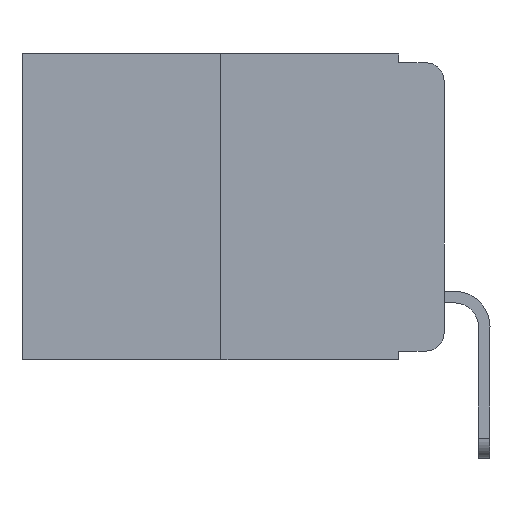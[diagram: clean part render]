
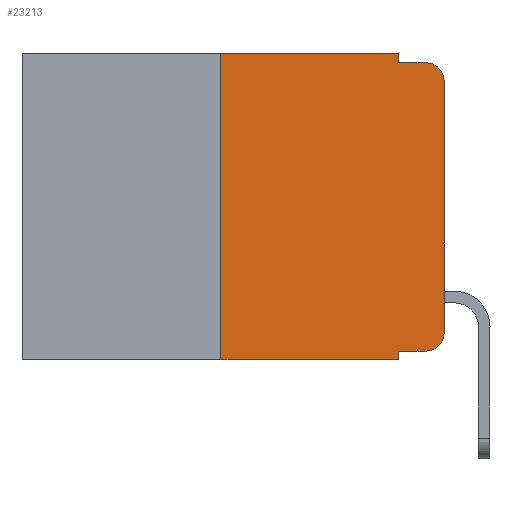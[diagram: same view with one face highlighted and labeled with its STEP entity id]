
A CAD part, left-side view. The second image highlights one B-rep face of the part: STEP entity #23213.
In plain terms, the highlighted planar face has unit normal (-1, 0, 0).
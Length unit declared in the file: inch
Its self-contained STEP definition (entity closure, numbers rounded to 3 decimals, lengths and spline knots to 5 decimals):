
#161 = EDGE_CURVE ( 'NONE', #10687, #3173, #15386, .T. ) ;
#646 = FACE_OUTER_BOUND ( 'NONE', #6226, .T. ) ;
#1108 = EDGE_CURVE ( 'NONE', #1517, #12400, #9660, .T. ) ;
#1128 = VECTOR ( 'NONE', #4296, 39.37008 ) ;
#1149 = CARTESIAN_POINT ( 'NONE',  ( 0., 0.051, -0.343 ) ) ;
#1398 = ORIENTED_EDGE ( 'NONE', *, *, #16433, .F. ) ;
#1502 = VERTEX_POINT ( 'NONE', #22279 ) ;
#1517 = VERTEX_POINT ( 'NONE', #6503 ) ;
#1681 = DIRECTION ( 'NONE',  ( 0., 0., -1. ) ) ;
#1985 = DIRECTION ( 'NONE',  ( -1., 0., 0. ) ) ;
#2085 = VERTEX_POINT ( 'NONE', #11511 ) ;
#2669 = VECTOR ( 'NONE', #2783, 39.37008 ) ;
#2783 = DIRECTION ( 'NONE',  ( 0., -1., 0. ) ) ;
#3173 = VERTEX_POINT ( 'NONE', #8655 ) ;
#3467 = DIRECTION ( 'NONE',  ( -1., 0., 0. ) ) ;
#3740 = DIRECTION ( 'NONE',  ( 0., 0., -1. ) ) ;
#3955 = DIRECTION ( 'NONE',  ( 0., 0., -1. ) ) ;
#4044 = VECTOR ( 'NONE', #16889, 39.37008 ) ;
#4296 = DIRECTION ( 'NONE',  ( 0., 0., 1. ) ) ;
#4309 = CARTESIAN_POINT ( 'NONE',  ( 0., 0.473, 0. ) ) ;
#4678 = ORIENTED_EDGE ( 'NONE', *, *, #1108, .F. ) ;
#5213 = EDGE_CURVE ( 'NONE', #1502, #2085, #18690, .T. ) ;
#5508 = CARTESIAN_POINT ( 'NONE',  ( 0., 0.25, 0. ) ) ;
#5619 = CARTESIAN_POINT ( 'NONE',  ( 0., 0.051, 0. ) ) ;
#6146 = EDGE_CURVE ( 'NONE', #22877, #2085, #9201, .T. ) ;
#6168 = LINE ( 'NONE', #9907, #1128 ) ;
#6214 = DIRECTION ( 'NONE',  ( 0., -1., 0. ) ) ;
#6226 = EDGE_LOOP ( 'NONE', ( #9166, #8071, #7068, #21740, #1398, #13635, #19643, #4678, #23053, #20347 ) ) ;
#6503 = CARTESIAN_POINT ( 'NONE',  ( 0., 0.051, -0.333 ) ) ;
#7068 = ORIENTED_EDGE ( 'NONE', *, *, #5213, .F. ) ;
#7911 = CARTESIAN_POINT ( 'NONE',  ( 0., 0.02, -0.03 ) ) ;
#8071 = ORIENTED_EDGE ( 'NONE', *, *, #6146, .T. ) ;
#8226 = VECTOR ( 'NONE', #3955, 39.37008 ) ;
#8655 = CARTESIAN_POINT ( 'NONE',  ( 0., 0., -0.313 ) ) ;
#8739 = AXIS2_PLACEMENT_3D ( 'NONE', #7911, #1985, #22385 ) ;
#8881 = EDGE_CURVE ( 'NONE', #20380, #1502, #22659, .T. ) ;
#8988 = CARTESIAN_POINT ( 'NONE',  ( 0., 0.02, -0.333 ) ) ;
#9090 = LINE ( 'NONE', #5508, #4044 ) ;
#9166 = ORIENTED_EDGE ( 'NONE', *, *, #18888, .T. ) ;
#9201 = CIRCLE ( 'NONE', #8739, 0.02 ) ;
#9660 = LINE ( 'NONE', #5619, #19158 ) ;
#9907 = CARTESIAN_POINT ( 'NONE',  ( 0., 0., 0. ) ) ;
#10687 = VERTEX_POINT ( 'NONE', #8988 ) ;
#10831 = CARTESIAN_POINT ( 'NONE',  ( 0., 0.051, 0. ) ) ;
#11511 = CARTESIAN_POINT ( 'NONE',  ( 0., 0.02, -0.01 ) ) ;
#11902 = VECTOR ( 'NONE', #14955, 39.37008 ) ;
#12200 = CARTESIAN_POINT ( 'NONE',  ( 0., 0., -0.03 ) ) ;
#12400 = VERTEX_POINT ( 'NONE', #1149 ) ;
#12491 = LINE ( 'NONE', #20552, #11902 ) ;
#12968 = LINE ( 'NONE', #4309, #17185 ) ;
#13206 = CARTESIAN_POINT ( 'NONE',  ( 0., 0.473, 0. ) ) ;
#13635 = ORIENTED_EDGE ( 'NONE', *, *, #17399, .F. ) ;
#13965 = CARTESIAN_POINT ( 'NONE',  ( 0., 0.051, -0.01 ) ) ;
#14134 = CARTESIAN_POINT ( 'NONE',  ( 0., 0.051, -0.333 ) ) ;
#14376 = CARTESIAN_POINT ( 'NONE',  ( 0., 0.02, -0.313 ) ) ;
#14655 = VERTEX_POINT ( 'NONE', #17230 ) ;
#14795 = DIRECTION ( 'NONE',  ( 0., 0., -1. ) ) ;
#14869 = EDGE_CURVE ( 'NONE', #1517, #10687, #21584, .T. ) ;
#14955 = DIRECTION ( 'NONE',  ( 0., -1., 0. ) ) ;
#15125 = DIRECTION ( 'NONE',  ( 1., 0., 0. ) ) ;
#15386 = CIRCLE ( 'NONE', #15913, 0.02 ) ;
#15913 = AXIS2_PLACEMENT_3D ( 'NONE', #14376, #3467, #1681 ) ;
#16433 = EDGE_CURVE ( 'NONE', #14655, #20380, #12968, .T. ) ;
#16889 = DIRECTION ( 'NONE',  ( 0., 0., 1. ) ) ;
#17185 = VECTOR ( 'NONE', #6214, 39.37008 ) ;
#17230 = CARTESIAN_POINT ( 'NONE',  ( 0., 0.25, 0. ) ) ;
#17399 = EDGE_CURVE ( 'NONE', #19374, #14655, #9090, .T. ) ;
#17556 = CARTESIAN_POINT ( 'NONE',  ( 0., 0.25, -0.343 ) ) ;
#18690 = LINE ( 'NONE', #13965, #21877 ) ;
#18888 = EDGE_CURVE ( 'NONE', #3173, #22877, #6168, .T. ) ;
#19118 = CARTESIAN_POINT ( 'NONE',  ( 0., 0.051, 0. ) ) ;
#19158 = VECTOR ( 'NONE', #14795, 39.37008 ) ;
#19374 = VERTEX_POINT ( 'NONE', #17556 ) ;
#19643 = ORIENTED_EDGE ( 'NONE', *, *, #23154, .T. ) ;
#20347 = ORIENTED_EDGE ( 'NONE', *, *, #161, .T. ) ;
#20380 = VERTEX_POINT ( 'NONE', #10831 ) ;
#20552 = CARTESIAN_POINT ( 'NONE',  ( 0., 0.473, -0.343 ) ) ;
#21584 = LINE ( 'NONE', #14134, #2669 ) ;
#21740 = ORIENTED_EDGE ( 'NONE', *, *, #8881, .F. ) ;
#21877 = VECTOR ( 'NONE', #23799, 39.37008 ) ;
#22279 = CARTESIAN_POINT ( 'NONE',  ( 0., 0.051, -0.01 ) ) ;
#22385 = DIRECTION ( 'NONE',  ( 0., 0., -1. ) ) ;
#22659 = LINE ( 'NONE', #19118, #8226 ) ;
#22877 = VERTEX_POINT ( 'NONE', #12200 ) ;
#23053 = ORIENTED_EDGE ( 'NONE', *, *, #14869, .T. ) ;
#23154 = EDGE_CURVE ( 'NONE', #19374, #12400, #12491, .T. ) ;
#23213 = ADVANCED_FACE ( 'NONE', ( #646 ), #24382, .F. ) ;
#23799 = DIRECTION ( 'NONE',  ( 0., -1., 0. ) ) ;
#23842 = AXIS2_PLACEMENT_3D ( 'NONE', #13206, #15125, #3740 ) ;
#24382 = PLANE ( 'NONE',  #23842 ) ;
